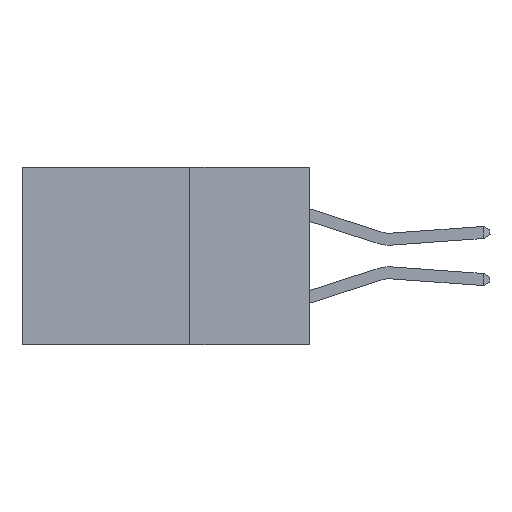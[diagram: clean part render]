
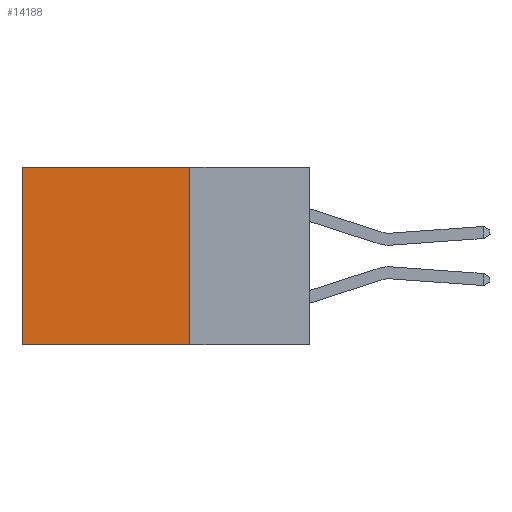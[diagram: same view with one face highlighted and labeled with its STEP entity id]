
A CAD part, left-side view. The second image highlights one B-rep face of the part: STEP entity #14188.
In plain terms, the highlighted planar face has unit normal (-1, 0, 0).
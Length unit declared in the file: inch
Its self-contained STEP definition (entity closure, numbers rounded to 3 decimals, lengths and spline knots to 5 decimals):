
#365 = DIRECTION ( 'NONE',  ( 1., 0., 0. ) ) ;
#1518 = CARTESIAN_POINT ( 'NONE',  ( 0.2615, 0.6, 0. ) ) ;
#2052 = VECTOR ( 'NONE', #4423, 39.37008 ) ;
#3873 = DIRECTION ( 'NONE',  ( 0., 0., -1. ) ) ;
#3990 = DIRECTION ( 'NONE',  ( 0., 0., -1. ) ) ;
#4348 = CARTESIAN_POINT ( 'NONE',  ( 0.2615, 0.25, -0.37 ) ) ;
#4423 = DIRECTION ( 'NONE',  ( 0., 1., 0. ) ) ;
#5218 = EDGE_CURVE ( 'NONE', #17493, #10970, #13542, .T. ) ;
#5386 = VERTEX_POINT ( 'NONE', #7413 ) ;
#5603 = LINE ( 'NONE', #10632, #16893 ) ;
#7413 = CARTESIAN_POINT ( 'NONE',  ( 0.2615, 0.25, 0. ) ) ;
#10632 = CARTESIAN_POINT ( 'NONE',  ( 0.2615, 0.25, -0.37 ) ) ;
#10687 = AXIS2_PLACEMENT_3D ( 'NONE', #4348, #365, #3990 ) ;
#10970 = VERTEX_POINT ( 'NONE', #15674 ) ;
#11127 = ORIENTED_EDGE ( 'NONE', *, *, #20910, .F. ) ;
#11533 = PLANE ( 'NONE',  #10687 ) ;
#12565 = DIRECTION ( 'NONE',  ( 0., 0., -1. ) ) ;
#12597 = LINE ( 'NONE', #19899, #13028 ) ;
#12779 = EDGE_CURVE ( 'NONE', #15897, #10970, #18259, .T. ) ;
#12804 = EDGE_LOOP ( 'NONE', ( #15820, #17047, #11127, #18501 ) ) ;
#13028 = VECTOR ( 'NONE', #14756, 39.37008 ) ;
#13542 = LINE ( 'NONE', #20840, #2052 ) ;
#14188 = ADVANCED_FACE ( 'NONE', ( #20409 ), #11533, .F. ) ;
#14756 = DIRECTION ( 'NONE',  ( 0., 1., 0. ) ) ;
#15194 = CARTESIAN_POINT ( 'NONE',  ( 0.2615, 0.25, -0.37 ) ) ;
#15313 = EDGE_CURVE ( 'NONE', #5386, #15897, #12597, .T. ) ;
#15674 = CARTESIAN_POINT ( 'NONE',  ( 0.2615, 0.6, -0.37 ) ) ;
#15820 = ORIENTED_EDGE ( 'NONE', *, *, #12779, .T. ) ;
#15897 = VERTEX_POINT ( 'NONE', #1518 ) ;
#16893 = VECTOR ( 'NONE', #12565, 39.37008 ) ;
#17047 = ORIENTED_EDGE ( 'NONE', *, *, #5218, .F. ) ;
#17166 = VECTOR ( 'NONE', #3873, 39.37008 ) ;
#17493 = VERTEX_POINT ( 'NONE', #15194 ) ;
#18259 = LINE ( 'NONE', #21611, #17166 ) ;
#18501 = ORIENTED_EDGE ( 'NONE', *, *, #15313, .T. ) ;
#19899 = CARTESIAN_POINT ( 'NONE',  ( 0.2615, 0.25, 0. ) ) ;
#20409 = FACE_OUTER_BOUND ( 'NONE', #12804, .T. ) ;
#20840 = CARTESIAN_POINT ( 'NONE',  ( 0.2615, 0.25, -0.37 ) ) ;
#20910 = EDGE_CURVE ( 'NONE', #5386, #17493, #5603, .T. ) ;
#21611 = CARTESIAN_POINT ( 'NONE',  ( 0.2615, 0.6, -0.37 ) ) ;
